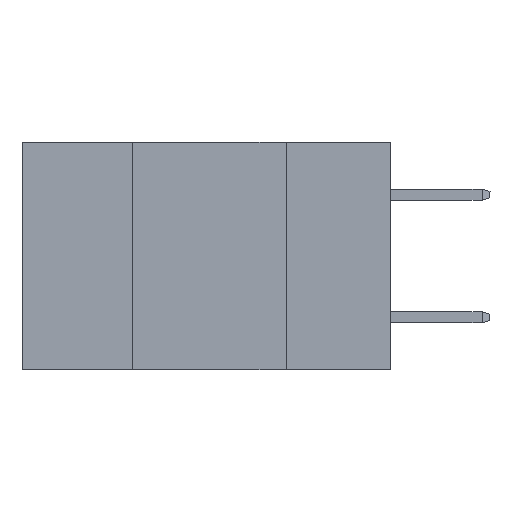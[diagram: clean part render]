
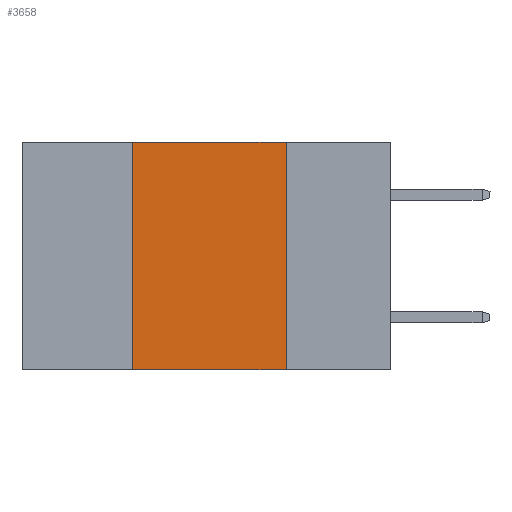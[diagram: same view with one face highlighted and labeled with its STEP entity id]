
A CAD part, left-side view. The second image highlights one B-rep face of the part: STEP entity #3658.
In plain terms, the highlighted planar face has unit normal (-1, 0, 0).
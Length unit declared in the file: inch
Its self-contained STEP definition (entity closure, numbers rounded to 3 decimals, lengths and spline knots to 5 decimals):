
#1816 = CARTESIAN_POINT ( 'NONE',  ( 0., 0.42, 0. ) ) ;
#3658 = ADVANCED_FACE ( 'NONE', ( #14911 ), #16033, .F. ) ;
#4366 = LINE ( 'NONE', #4531, #14977 ) ;
#4531 = CARTESIAN_POINT ( 'NONE',  ( 0., 0.17, 0. ) ) ;
#4553 = CARTESIAN_POINT ( 'NONE',  ( 0., 0.6, 0. ) ) ;
#4647 = LINE ( 'NONE', #4553, #17415 ) ;
#5034 = DIRECTION ( 'NONE',  ( 0., 0., 1. ) ) ;
#5243 = EDGE_CURVE ( 'NONE', #19821, #15333, #21115, .T. ) ;
#6321 = AXIS2_PLACEMENT_3D ( 'NONE', #16114, #16316, #16911 ) ;
#7226 = VERTEX_POINT ( 'NONE', #14388 ) ;
#7652 = ORIENTED_EDGE ( 'NONE', *, *, #9743, .T. ) ;
#9569 = DIRECTION ( 'NONE',  ( 0., -1., 0. ) ) ;
#9743 = EDGE_CURVE ( 'NONE', #19821, #7226, #15796, .T. ) ;
#11147 = CARTESIAN_POINT ( 'NONE',  ( 0., 0.42, 0. ) ) ;
#11898 = VECTOR ( 'NONE', #14287, 39.37008 ) ;
#13089 = CARTESIAN_POINT ( 'NONE',  ( 0., 0.42, -0.37 ) ) ;
#13817 = ORIENTED_EDGE ( 'NONE', *, *, #20366, .F. ) ;
#13915 = EDGE_LOOP ( 'NONE', ( #13817, #16653, #14358, #7652 ) ) ;
#14287 = DIRECTION ( 'NONE',  ( 0., -1., 0. ) ) ;
#14358 = ORIENTED_EDGE ( 'NONE', *, *, #5243, .F. ) ;
#14388 = CARTESIAN_POINT ( 'NONE',  ( 0., 0.17, -0.37 ) ) ;
#14460 = DIRECTION ( 'NONE',  ( 0., 0., -1. ) ) ;
#14911 = FACE_OUTER_BOUND ( 'NONE', #13915, .T. ) ;
#14977 = VECTOR ( 'NONE', #14460, 39.37008 ) ;
#15333 = VERTEX_POINT ( 'NONE', #11147 ) ;
#15796 = LINE ( 'NONE', #15964, #11898 ) ;
#15964 = CARTESIAN_POINT ( 'NONE',  ( 0., 0.6, -0.37 ) ) ;
#16033 = PLANE ( 'NONE',  #6321 ) ;
#16114 = CARTESIAN_POINT ( 'NONE',  ( 0., 0.6, 0. ) ) ;
#16190 = VECTOR ( 'NONE', #5034, 39.37008 ) ;
#16316 = DIRECTION ( 'NONE',  ( 1., 0., 0. ) ) ;
#16653 = ORIENTED_EDGE ( 'NONE', *, *, #19732, .F. ) ;
#16911 = DIRECTION ( 'NONE',  ( 0., 0., -1. ) ) ;
#17415 = VECTOR ( 'NONE', #9569, 39.37008 ) ;
#17567 = CARTESIAN_POINT ( 'NONE',  ( 0., 0.17, 0. ) ) ;
#19732 = EDGE_CURVE ( 'NONE', #15333, #20248, #4647, .T. ) ;
#19821 = VERTEX_POINT ( 'NONE', #13089 ) ;
#20248 = VERTEX_POINT ( 'NONE', #17567 ) ;
#20366 = EDGE_CURVE ( 'NONE', #20248, #7226, #4366, .T. ) ;
#21115 = LINE ( 'NONE', #1816, #16190 ) ;
